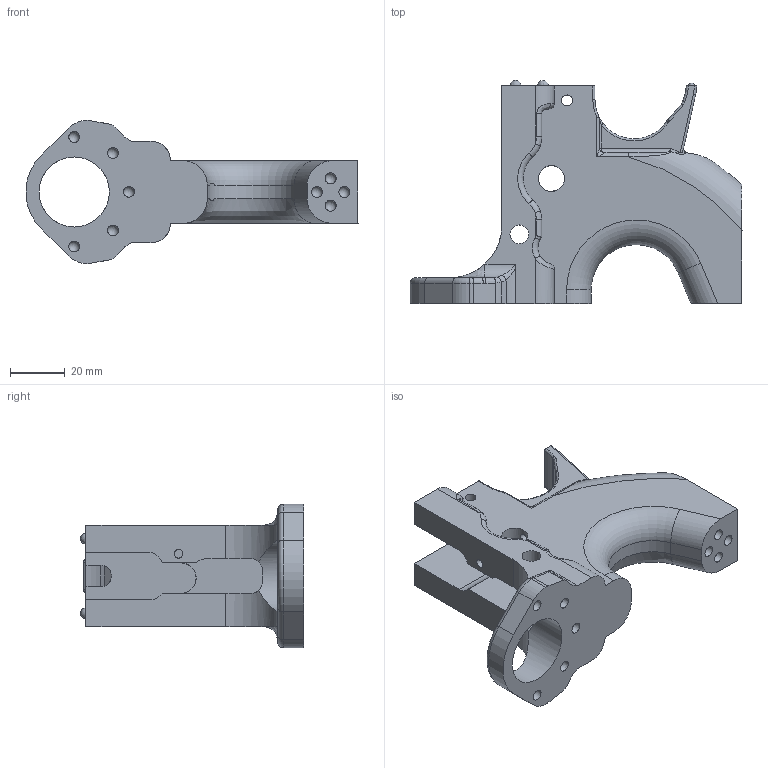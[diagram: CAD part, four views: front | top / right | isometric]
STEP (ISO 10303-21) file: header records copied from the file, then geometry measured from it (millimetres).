
FILE_DESCRIPTION (( 'STEP AP214' ), '1' );
FILE_NAME ('Atlas_SSR_Receiver_Rear_V2.step', '2016-01-25T18:17:08', ( 'WarFairy' ), ( '' ), 'SwSTEP 2.0', 'SolidWorks 2015', '' );
FILE_SCHEMA (( 'AUTOMOTIVE_DESIGN' ));
Length unit declared in the file: millimetre
Products named in the file (1): Atlas_SSR_Receiver_Rear_V2
Bounding box: 121.38 x 81.54 x 52.5 mm (x, y, z)
Volume: 117307.9 mm3; surface area: 27697.7 mm2
Topology: 1 solids, 1 shells, 237 faces, 660 edges, 399 vertices
Faces by surface type: cylinder 91, bspline 62, plane 46, torus 23, sphere 15
Full cylindrical faces by diameter (mm): 3.175 x2, 3.969 x2, 6.858 x2, 9.525 x2, 25.654 x1
Entity records: 10842 total; most frequent: CARTESIAN_POINT 5537, ORIENTED_EDGE 1176, DIRECTION 993, EDGE_CURVE 588, AXIS2_PLACEMENT_3D 396, VERTEX_POINT 374, EDGE_LOOP 274, FACE_OUTER_BOUND 246
